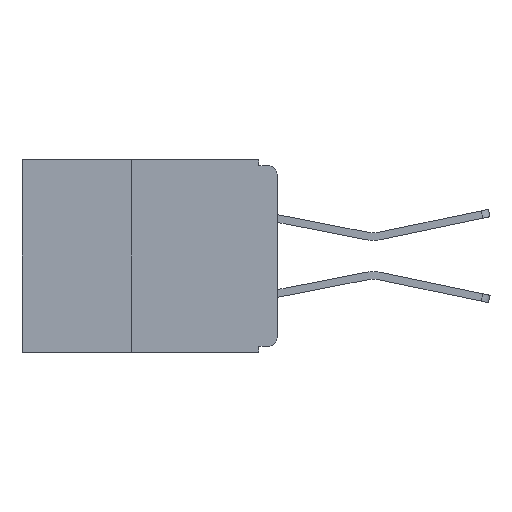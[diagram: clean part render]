
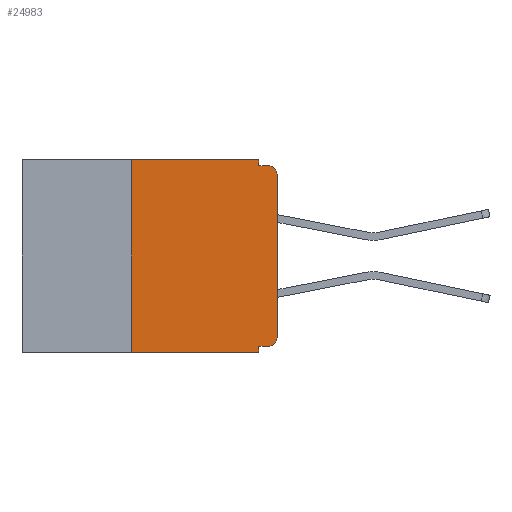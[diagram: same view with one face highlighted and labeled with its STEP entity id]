
A CAD part, left-side view. The second image highlights one B-rep face of the part: STEP entity #24983.
In plain terms, the highlighted planar face has unit normal (-1, 0, 0).
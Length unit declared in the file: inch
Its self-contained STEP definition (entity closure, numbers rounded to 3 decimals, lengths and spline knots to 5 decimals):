
#104 = EDGE_CURVE ( 'NONE', #23691, #15218, #6831, .T. ) ;
#547 = ORIENTED_EDGE ( 'NONE', *, *, #18966, .T. ) ;
#658 = CIRCLE ( 'NONE', #27570, 0.015 ) ;
#1883 = VERTEX_POINT ( 'NONE', #24462 ) ;
#2061 = CARTESIAN_POINT ( 'NONE',  ( 0., 0.25, -0.33 ) ) ;
#3230 = VERTEX_POINT ( 'NONE', #30594 ) ;
#4168 = DIRECTION ( 'NONE',  ( 0., 0., -1. ) ) ;
#5431 = LINE ( 'NONE', #33457, #32285 ) ;
#5473 = EDGE_LOOP ( 'NONE', ( #28756, #23560, #24359, #31968, #25983, #20742, #547, #8423, #29170, #29979 ) ) ;
#6337 = CARTESIAN_POINT ( 'NONE',  ( 0., 0.031, -0.33 ) ) ;
#6831 = CIRCLE ( 'NONE', #13159, 0.015 ) ;
#6923 = VERTEX_POINT ( 'NONE', #13211 ) ;
#7234 = CARTESIAN_POINT ( 'NONE',  ( 0., 0.031, 0. ) ) ;
#8226 = VERTEX_POINT ( 'NONE', #2061 ) ;
#8423 = ORIENTED_EDGE ( 'NONE', *, *, #8456, .F. ) ;
#8456 = EDGE_CURVE ( 'NONE', #6923, #16568, #8750, .T. ) ;
#8733 = CARTESIAN_POINT ( 'NONE',  ( 0., 0.437, -0.33 ) ) ;
#8750 = LINE ( 'NONE', #26184, #15718 ) ;
#8915 = DIRECTION ( 'NONE',  ( 0., 0., 1. ) ) ;
#9330 = CARTESIAN_POINT ( 'NONE',  ( 0., 0., -0.32 ) ) ;
#9396 = VECTOR ( 'NONE', #30099, 39.37008 ) ;
#9410 = CARTESIAN_POINT ( 'NONE',  ( 0., 0.437, 0. ) ) ;
#9643 = DIRECTION ( 'NONE',  ( 0., 0., -1. ) ) ;
#11410 = CARTESIAN_POINT ( 'NONE',  ( 0., 0.015, -0.01 ) ) ;
#12443 = LINE ( 'NONE', #25282, #26286 ) ;
#12645 = DIRECTION ( 'NONE',  ( -1., 0., 0. ) ) ;
#13081 = EDGE_CURVE ( 'NONE', #22666, #6923, #23285, .T. ) ;
#13136 = LINE ( 'NONE', #8733, #26168 ) ;
#13159 = AXIS2_PLACEMENT_3D ( 'NONE', #21727, #21997, #24798 ) ;
#13211 = CARTESIAN_POINT ( 'NONE',  ( 0., 0.031, -0.32 ) ) ;
#14480 = FACE_OUTER_BOUND ( 'NONE', #5473, .T. ) ;
#15218 = VERTEX_POINT ( 'NONE', #11410 ) ;
#15718 = VECTOR ( 'NONE', #26606, 39.37008 ) ;
#15950 = CARTESIAN_POINT ( 'NONE',  ( 0., 0.015, -0.32 ) ) ;
#16343 = DIRECTION ( 'NONE',  ( 0., -1., 0. ) ) ;
#16408 = CARTESIAN_POINT ( 'NONE',  ( 0., 0., 0. ) ) ;
#16568 = VERTEX_POINT ( 'NONE', #6337 ) ;
#17434 = AXIS2_PLACEMENT_3D ( 'NONE', #9410, #19940, #4168 ) ;
#18085 = CARTESIAN_POINT ( 'NONE',  ( 0., 0., -0.025 ) ) ;
#18265 = EDGE_CURVE ( 'NONE', #3230, #15218, #20913, .T. ) ;
#18614 = VERTEX_POINT ( 'NONE', #7234 ) ;
#18966 = EDGE_CURVE ( 'NONE', #8226, #16568, #13136, .T. ) ;
#19053 = DIRECTION ( 'NONE',  ( 0., 0., 1. ) ) ;
#19345 = CARTESIAN_POINT ( 'NONE',  ( 0., 0.25, -0.33 ) ) ;
#19940 = DIRECTION ( 'NONE',  ( 1., 0., 0. ) ) ;
#20742 = ORIENTED_EDGE ( 'NONE', *, *, #25514, .F. ) ;
#20913 = LINE ( 'NONE', #31813, #26961 ) ;
#21727 = CARTESIAN_POINT ( 'NONE',  ( 0., 0.015, -0.025 ) ) ;
#21927 = VECTOR ( 'NONE', #19053, 39.37008 ) ;
#21997 = DIRECTION ( 'NONE',  ( -1., 0., 0. ) ) ;
#22666 = VERTEX_POINT ( 'NONE', #15950 ) ;
#22732 = LINE ( 'NONE', #16408, #21927 ) ;
#23285 = LINE ( 'NONE', #9330, #9396 ) ;
#23560 = ORIENTED_EDGE ( 'NONE', *, *, #104, .T. ) ;
#23691 = VERTEX_POINT ( 'NONE', #18085 ) ;
#23695 = EDGE_CURVE ( 'NONE', #26071, #18614, #5431, .T. ) ;
#24359 = ORIENTED_EDGE ( 'NONE', *, *, #18265, .F. ) ;
#24462 = CARTESIAN_POINT ( 'NONE',  ( 0., 0., -0.305 ) ) ;
#24798 = DIRECTION ( 'NONE',  ( 0., 0., -1. ) ) ;
#24816 = EDGE_CURVE ( 'NONE', #18614, #3230, #12443, .T. ) ;
#24983 = ADVANCED_FACE ( 'NONE', ( #14480 ), #30182, .F. ) ;
#25282 = CARTESIAN_POINT ( 'NONE',  ( 0., 0.031, 0. ) ) ;
#25514 = EDGE_CURVE ( 'NONE', #8226, #26071, #33396, .T. ) ;
#25901 = DIRECTION ( 'NONE',  ( 0., -1., 0. ) ) ;
#25983 = ORIENTED_EDGE ( 'NONE', *, *, #23695, .F. ) ;
#26071 = VERTEX_POINT ( 'NONE', #32116 ) ;
#26168 = VECTOR ( 'NONE', #29524, 39.37008 ) ;
#26184 = CARTESIAN_POINT ( 'NONE',  ( 0., 0.031, -0.33 ) ) ;
#26286 = VECTOR ( 'NONE', #9643, 39.37008 ) ;
#26606 = DIRECTION ( 'NONE',  ( 0., 0., -1. ) ) ;
#26653 = VECTOR ( 'NONE', #8915, 39.37008 ) ;
#26961 = VECTOR ( 'NONE', #16343, 39.37008 ) ;
#27570 = AXIS2_PLACEMENT_3D ( 'NONE', #28194, #12645, #30780 ) ;
#27852 = EDGE_CURVE ( 'NONE', #1883, #23691, #22732, .T. ) ;
#28194 = CARTESIAN_POINT ( 'NONE',  ( 0., 0.015, -0.305 ) ) ;
#28756 = ORIENTED_EDGE ( 'NONE', *, *, #27852, .T. ) ;
#29170 = ORIENTED_EDGE ( 'NONE', *, *, #13081, .F. ) ;
#29524 = DIRECTION ( 'NONE',  ( 0., -1., 0. ) ) ;
#29979 = ORIENTED_EDGE ( 'NONE', *, *, #33573, .T. ) ;
#30099 = DIRECTION ( 'NONE',  ( 0., 1., 0. ) ) ;
#30182 = PLANE ( 'NONE',  #17434 ) ;
#30594 = CARTESIAN_POINT ( 'NONE',  ( 0., 0.031, -0.01 ) ) ;
#30780 = DIRECTION ( 'NONE',  ( 0., 0., -1. ) ) ;
#31813 = CARTESIAN_POINT ( 'NONE',  ( 0., 0., -0.01 ) ) ;
#31968 = ORIENTED_EDGE ( 'NONE', *, *, #24816, .F. ) ;
#32116 = CARTESIAN_POINT ( 'NONE',  ( 0., 0.25, 0. ) ) ;
#32285 = VECTOR ( 'NONE', #25901, 39.37008 ) ;
#33396 = LINE ( 'NONE', #19345, #26653 ) ;
#33457 = CARTESIAN_POINT ( 'NONE',  ( 0., 0.437, 0. ) ) ;
#33573 = EDGE_CURVE ( 'NONE', #22666, #1883, #658, .T. ) ;
